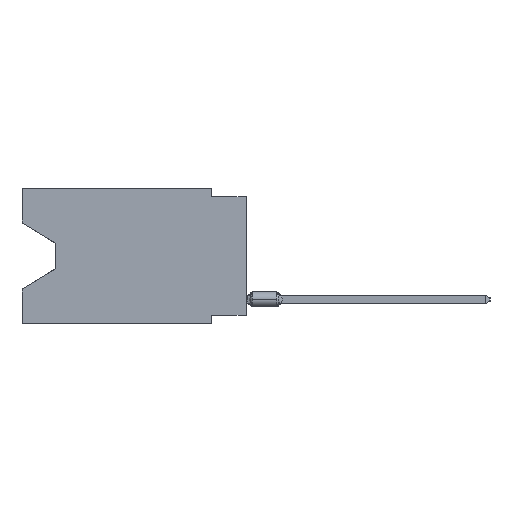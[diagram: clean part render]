
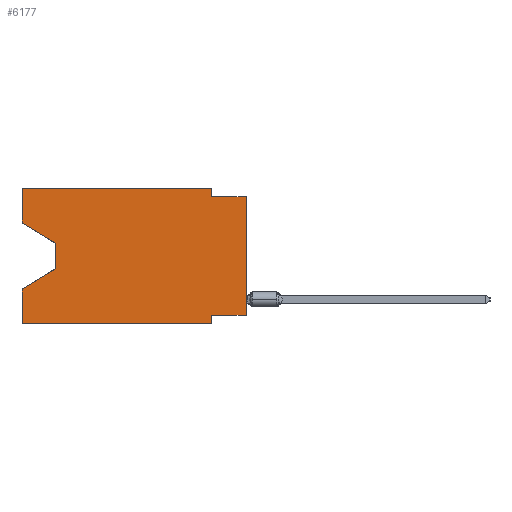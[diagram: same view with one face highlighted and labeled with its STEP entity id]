
A CAD part, left-side view. The second image highlights one B-rep face of the part: STEP entity #6177.
In plain terms, the highlighted planar face has unit normal (-1, 0, 0).
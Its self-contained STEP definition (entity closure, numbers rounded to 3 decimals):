
#191 = ORIENTED_EDGE ( 'NONE', *, *, #27706, .F. ) ;
#1217 = DIRECTION ( 'NONE',  ( 0., 0., 1. ) ) ;
#1408 = VECTOR ( 'NONE', #22464, 1000. ) ;
#1787 = DIRECTION ( 'NONE',  ( 0., 0., 1. ) ) ;
#1927 = VERTEX_POINT ( 'NONE', #26819 ) ;
#2616 = VERTEX_POINT ( 'NONE', #12460 ) ;
#3299 = CARTESIAN_POINT ( 'NONE',  ( 0., 16.383, 0. ) ) ;
#4136 = VERTEX_POINT ( 'NONE', #35140 ) ;
#4190 = EDGE_CURVE ( 'NONE', #16626, #18945, #25663, .T. ) ;
#4309 = EDGE_CURVE ( 'NONE', #53746, #2616, #53001, .T. ) ;
#5162 = VERTEX_POINT ( 'NONE', #51780 ) ;
#5373 = VECTOR ( 'NONE', #49276, 1000. ) ;
#5406 = CARTESIAN_POINT ( 'NONE',  ( 0., 16.383, 0. ) ) ;
#6177 = ADVANCED_FACE ( 'NONE', ( #32934 ), #33216, .F. ) ;
#6597 = DIRECTION ( 'NONE',  ( 0., 0., -1. ) ) ;
#6763 = CARTESIAN_POINT ( 'NONE',  ( 0., 16.383, 0. ) ) ;
#7282 = LINE ( 'NONE', #13679, #50733 ) ;
#7536 = CARTESIAN_POINT ( 'NONE',  ( 0., 16.383, -2.546 ) ) ;
#7821 = VECTOR ( 'NONE', #36686, 1000. ) ;
#8025 = ORIENTED_EDGE ( 'NONE', *, *, #26090, .F. ) ;
#8059 = VECTOR ( 'NONE', #48768, 1000. ) ;
#8544 = LINE ( 'NONE', #39305, #54120 ) ;
#9110 = VERTEX_POINT ( 'NONE', #3299 ) ;
#10006 = VECTOR ( 'NONE', #17526, 1000. ) ;
#10248 = CARTESIAN_POINT ( 'NONE',  ( 0., 2.54, 0. ) ) ;
#12288 = VECTOR ( 'NONE', #14390, 1000. ) ;
#12460 = CARTESIAN_POINT ( 'NONE',  ( 0., 2.54, -0.635 ) ) ;
#13020 = DIRECTION ( 'NONE',  ( 0., -1., 0. ) ) ;
#13679 = CARTESIAN_POINT ( 'NONE',  ( 0., 13.97, -5.893 ) ) ;
#14390 = DIRECTION ( 'NONE',  ( 0., 0., -1. ) ) ;
#15112 = ORIENTED_EDGE ( 'NONE', *, *, #26164, .T. ) ;
#16047 = EDGE_CURVE ( 'NONE', #5162, #36682, #7282, .T. ) ;
#16626 = VERTEX_POINT ( 'NONE', #7536 ) ;
#17526 = DIRECTION ( 'NONE',  ( 0., -0.855, -0.519 ) ) ;
#18303 = VERTEX_POINT ( 'NONE', #22199 ) ;
#18413 = EDGE_CURVE ( 'NONE', #18945, #5162, #23011, .T. ) ;
#18462 = EDGE_CURVE ( 'NONE', #16626, #9110, #19349, .T. ) ;
#18595 = CARTESIAN_POINT ( 'NONE',  ( 0., 0., -0.635 ) ) ;
#18728 = EDGE_CURVE ( 'NONE', #2616, #1927, #39844, .T. ) ;
#18831 = LINE ( 'NONE', #26673, #37719 ) ;
#18945 = VERTEX_POINT ( 'NONE', #36959 ) ;
#19258 = CARTESIAN_POINT ( 'NONE',  ( 0., 16.383, -9.906 ) ) ;
#19349 = LINE ( 'NONE', #6763, #49094 ) ;
#19535 = ORIENTED_EDGE ( 'NONE', *, *, #18462, .F. ) ;
#19633 = LINE ( 'NONE', #23815, #7821 ) ;
#21519 = DIRECTION ( 'NONE',  ( 0., 0.855, -0.519 ) ) ;
#22199 = CARTESIAN_POINT ( 'NONE',  ( 0., 2.54, -9.906 ) ) ;
#22464 = DIRECTION ( 'NONE',  ( 0., -1., 0. ) ) ;
#22760 = LINE ( 'NONE', #35338, #12288 ) ;
#23011 = LINE ( 'NONE', #23290, #5373 ) ;
#23290 = CARTESIAN_POINT ( 'NONE',  ( 0., 13.97, -4.013 ) ) ;
#23815 = CARTESIAN_POINT ( 'NONE',  ( 0., 0., -9.271 ) ) ;
#24146 = EDGE_LOOP ( 'NONE', ( #45335, #53820, #40330, #29153, #15112, #191, #8025, #40476, #27676, #33850, #34462, #19535 ) ) ;
#25206 = VERTEX_POINT ( 'NONE', #39715 ) ;
#25663 = LINE ( 'NONE', #42717, #10006 ) ;
#26090 = EDGE_CURVE ( 'NONE', #4136, #25206, #19633, .T. ) ;
#26164 = EDGE_CURVE ( 'NONE', #28140, #18303, #8544, .T. ) ;
#26673 = CARTESIAN_POINT ( 'NONE',  ( 0., 16.383, 0. ) ) ;
#26819 = CARTESIAN_POINT ( 'NONE',  ( 0., 0., -0.635 ) ) ;
#27676 = ORIENTED_EDGE ( 'NONE', *, *, #18728, .F. ) ;
#27706 = EDGE_CURVE ( 'NONE', #25206, #18303, #22760, .T. ) ;
#28140 = VERTEX_POINT ( 'NONE', #19258 ) ;
#29153 = ORIENTED_EDGE ( 'NONE', *, *, #39464, .F. ) ;
#29805 = LINE ( 'NONE', #46860, #54927 ) ;
#30103 = EDGE_CURVE ( 'NONE', #4136, #1927, #29805, .T. ) ;
#31913 = LINE ( 'NONE', #5406, #1408 ) ;
#32934 = FACE_OUTER_BOUND ( 'NONE', #24146, .T. ) ;
#33080 = DIRECTION ( 'NONE',  ( 0., 0., 1. ) ) ;
#33216 = PLANE ( 'NONE',  #47639 ) ;
#33850 = ORIENTED_EDGE ( 'NONE', *, *, #4309, .F. ) ;
#34462 = ORIENTED_EDGE ( 'NONE', *, *, #54359, .F. ) ;
#35140 = CARTESIAN_POINT ( 'NONE',  ( 0., 0., -9.271 ) ) ;
#35338 = CARTESIAN_POINT ( 'NONE',  ( 0., 2.54, -9.906 ) ) ;
#36682 = VERTEX_POINT ( 'NONE', #38693 ) ;
#36686 = DIRECTION ( 'NONE',  ( 0., 1., 0. ) ) ;
#36959 = CARTESIAN_POINT ( 'NONE',  ( 0., 13.97, -4.013 ) ) ;
#37719 = VECTOR ( 'NONE', #1787, 1000. ) ;
#38693 = CARTESIAN_POINT ( 'NONE',  ( 0., 16.383, -7.36 ) ) ;
#39305 = CARTESIAN_POINT ( 'NONE',  ( 0., 16.383, -9.906 ) ) ;
#39464 = EDGE_CURVE ( 'NONE', #28140, #36682, #18831, .T. ) ;
#39715 = CARTESIAN_POINT ( 'NONE',  ( 0., 2.54, -9.271 ) ) ;
#39844 = LINE ( 'NONE', #18595, #8059 ) ;
#40330 = ORIENTED_EDGE ( 'NONE', *, *, #16047, .T. ) ;
#40476 = ORIENTED_EDGE ( 'NONE', *, *, #30103, .T. ) ;
#42717 = CARTESIAN_POINT ( 'NONE',  ( 0., 16.383, -2.546 ) ) ;
#44833 = VECTOR ( 'NONE', #6597, 1000. ) ;
#45335 = ORIENTED_EDGE ( 'NONE', *, *, #4190, .T. ) ;
#45496 = CARTESIAN_POINT ( 'NONE',  ( 0., 2.54, 0. ) ) ;
#46073 = DIRECTION ( 'NONE',  ( 1., 0., 0. ) ) ;
#46860 = CARTESIAN_POINT ( 'NONE',  ( 0., 0., 0. ) ) ;
#47639 = AXIS2_PLACEMENT_3D ( 'NONE', #49992, #46073, #54467 ) ;
#48768 = DIRECTION ( 'NONE',  ( 0., -1., 0. ) ) ;
#49094 = VECTOR ( 'NONE', #1217, 1000. ) ;
#49276 = DIRECTION ( 'NONE',  ( 0., 0., -1. ) ) ;
#49992 = CARTESIAN_POINT ( 'NONE',  ( 0., 16.383, 0. ) ) ;
#50733 = VECTOR ( 'NONE', #21519, 1000. ) ;
#51780 = CARTESIAN_POINT ( 'NONE',  ( 0., 13.97, -5.893 ) ) ;
#53001 = LINE ( 'NONE', #10248, #44833 ) ;
#53746 = VERTEX_POINT ( 'NONE', #45496 ) ;
#53820 = ORIENTED_EDGE ( 'NONE', *, *, #18413, .T. ) ;
#54120 = VECTOR ( 'NONE', #13020, 1000. ) ;
#54359 = EDGE_CURVE ( 'NONE', #9110, #53746, #31913, .T. ) ;
#54467 = DIRECTION ( 'NONE',  ( 0., 0., -1. ) ) ;
#54927 = VECTOR ( 'NONE', #33080, 1000. ) ;
